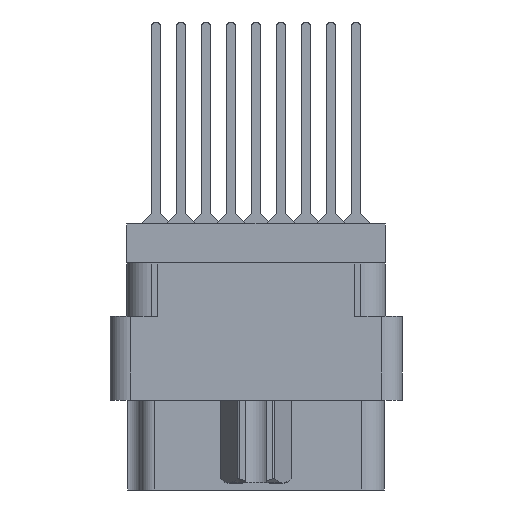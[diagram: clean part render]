
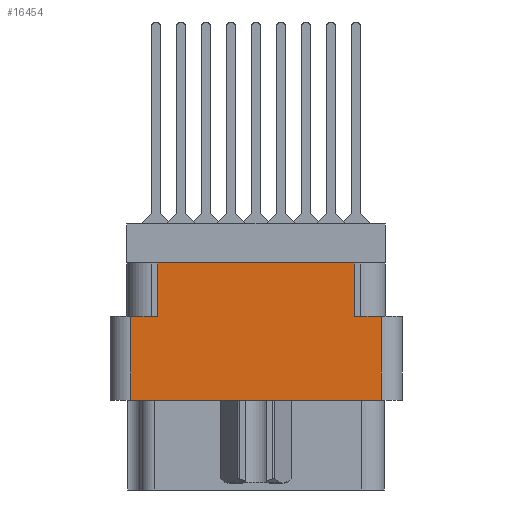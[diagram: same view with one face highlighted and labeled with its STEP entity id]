
A CAD part, left-side view. The second image highlights one B-rep face of the part: STEP entity #16454.
In plain terms, the highlighted planar face has unit normal (-1, 0, 0).
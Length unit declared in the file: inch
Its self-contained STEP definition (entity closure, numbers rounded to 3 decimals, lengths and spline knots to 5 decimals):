
#899 = DIRECTION ( 'NONE',  ( 0., 0., 1. ) ) ;
#1416 = DIRECTION ( 'NONE',  ( 0., -1., 0. ) ) ;
#1868 = ORIENTED_EDGE ( 'NONE', *, *, #14493, .F. ) ;
#2333 = ORIENTED_EDGE ( 'NONE', *, *, #22572, .T. ) ;
#2398 = CARTESIAN_POINT ( 'NONE',  ( -1., 0., -0.277 ) ) ;
#3328 = EDGE_LOOP ( 'NONE', ( #1868, #12689, #12757, #7398, #14061, #2333, #43179, #23534 ) ) ;
#4419 = CARTESIAN_POINT ( 'NONE',  ( -1., 0.296, -0.277 ) ) ;
#5922 = VECTOR ( 'NONE', #35700, 39.37008 ) ;
#6975 = CARTESIAN_POINT ( 'NONE',  ( -1., 0.376, -0.277 ) ) ;
#7096 = LINE ( 'NONE', #10103, #5922 ) ;
#7398 = ORIENTED_EDGE ( 'NONE', *, *, #16178, .T. ) ;
#8435 = CARTESIAN_POINT ( 'NONE',  ( -1., -0.376, -0.277 ) ) ;
#8513 = CARTESIAN_POINT ( 'NONE',  ( -1., 0.438, -0.117 ) ) ;
#10103 = CARTESIAN_POINT ( 'NONE',  ( -1., -0.296, -0.277 ) ) ;
#10436 = CARTESIAN_POINT ( 'NONE',  ( -1., 0.296, -0.117 ) ) ;
#10806 = CARTESIAN_POINT ( 'NONE',  ( -1., -0.296, -0.277 ) ) ;
#11649 = VERTEX_POINT ( 'NONE', #17782 ) ;
#12088 = VECTOR ( 'NONE', #30104, 39.37008 ) ;
#12575 = EDGE_CURVE ( 'NONE', #46240, #26281, #19398, .T. ) ;
#12689 = ORIENTED_EDGE ( 'NONE', *, *, #45200, .T. ) ;
#12757 = ORIENTED_EDGE ( 'NONE', *, *, #12937, .F. ) ;
#12836 = FACE_OUTER_BOUND ( 'NONE', #3328, .T. ) ;
#12937 = EDGE_CURVE ( 'NONE', #38181, #11649, #42208, .T. ) ;
#14061 = ORIENTED_EDGE ( 'NONE', *, *, #16881, .F. ) ;
#14493 = EDGE_CURVE ( 'NONE', #18745, #45284, #46216, .T. ) ;
#14812 = LINE ( 'NONE', #25801, #37686 ) ;
#15076 = DIRECTION ( 'NONE',  ( 0., 1., 0. ) ) ;
#15689 = CARTESIAN_POINT ( 'NONE',  ( -1., 0.296, -0.277 ) ) ;
#15728 = DIRECTION ( 'NONE',  ( 0., -1., 0. ) ) ;
#15847 = VECTOR ( 'NONE', #35568, 39.37008 ) ;
#16178 = EDGE_CURVE ( 'NONE', #38181, #41446, #40353, .T. ) ;
#16454 = ADVANCED_FACE ( 'NONE', ( #12836 ), #46402, .T. ) ;
#16881 = EDGE_CURVE ( 'NONE', #29219, #41446, #32849, .T. ) ;
#17658 = VECTOR ( 'NONE', #15076, 39.37008 ) ;
#17702 = VECTOR ( 'NONE', #1416, 39.37008 ) ;
#17782 = CARTESIAN_POINT ( 'NONE',  ( -1., 0.376, -0.529 ) ) ;
#18108 = EDGE_CURVE ( 'NONE', #45284, #46240, #19557, .T. ) ;
#18745 = VERTEX_POINT ( 'NONE', #6975 ) ;
#19398 = LINE ( 'NONE', #8513, #17702 ) ;
#19557 = LINE ( 'NONE', #4419, #12088 ) ;
#20766 = DIRECTION ( 'NONE',  ( -1., 0., 0. ) ) ;
#20892 = VECTOR ( 'NONE', #899, 39.37008 ) ;
#20922 = CARTESIAN_POINT ( 'NONE',  ( -1., -0.438, -0.798 ) ) ;
#22572 = EDGE_CURVE ( 'NONE', #29219, #26281, #7096, .T. ) ;
#23534 = ORIENTED_EDGE ( 'NONE', *, *, #18108, .F. ) ;
#25796 = CARTESIAN_POINT ( 'NONE',  ( -1., 0., -0.529 ) ) ;
#25801 = CARTESIAN_POINT ( 'NONE',  ( -1., 0.376, -0.798 ) ) ;
#26281 = VERTEX_POINT ( 'NONE', #32751 ) ;
#26773 = CARTESIAN_POINT ( 'NONE',  ( -1., 0., -0.277 ) ) ;
#28612 = AXIS2_PLACEMENT_3D ( 'NONE', #20922, #20766, #31829 ) ;
#29219 = VERTEX_POINT ( 'NONE', #10806 ) ;
#29638 = DIRECTION ( 'NONE',  ( 0., 0., -1. ) ) ;
#30104 = DIRECTION ( 'NONE',  ( 0., 0., 1. ) ) ;
#31829 = DIRECTION ( 'NONE',  ( 0., 0., 1. ) ) ;
#32751 = CARTESIAN_POINT ( 'NONE',  ( -1., -0.296, -0.117 ) ) ;
#32849 = LINE ( 'NONE', #26773, #36861 ) ;
#35568 = DIRECTION ( 'NONE',  ( 0., -1., 0. ) ) ;
#35700 = DIRECTION ( 'NONE',  ( 0., 0., 1. ) ) ;
#36861 = VECTOR ( 'NONE', #15728, 39.37008 ) ;
#37686 = VECTOR ( 'NONE', #29638, 39.37008 ) ;
#38181 = VERTEX_POINT ( 'NONE', #44645 ) ;
#40353 = LINE ( 'NONE', #41406, #20892 ) ;
#41406 = CARTESIAN_POINT ( 'NONE',  ( -1., -0.376, -0.798 ) ) ;
#41446 = VERTEX_POINT ( 'NONE', #8435 ) ;
#42208 = LINE ( 'NONE', #25796, #17658 ) ;
#43179 = ORIENTED_EDGE ( 'NONE', *, *, #12575, .F. ) ;
#44645 = CARTESIAN_POINT ( 'NONE',  ( -1., -0.376, -0.529 ) ) ;
#45200 = EDGE_CURVE ( 'NONE', #18745, #11649, #14812, .T. ) ;
#45284 = VERTEX_POINT ( 'NONE', #15689 ) ;
#46216 = LINE ( 'NONE', #2398, #15847 ) ;
#46240 = VERTEX_POINT ( 'NONE', #10436 ) ;
#46402 = PLANE ( 'NONE',  #28612 ) ;
